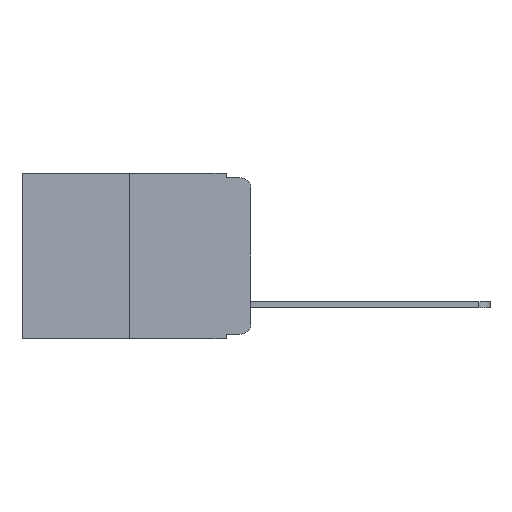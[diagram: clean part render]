
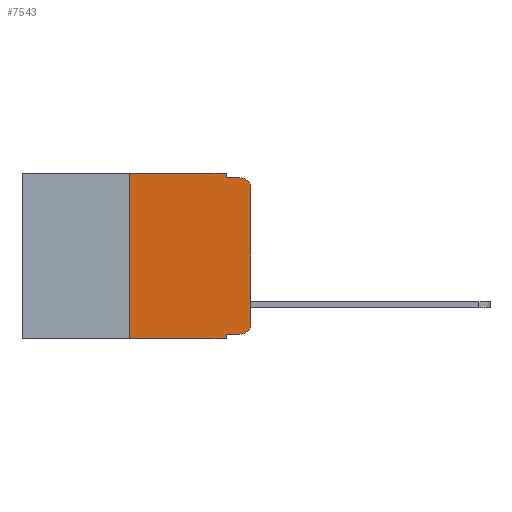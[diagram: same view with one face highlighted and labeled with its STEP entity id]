
A CAD part, left-side view. The second image highlights one B-rep face of the part: STEP entity #7543.
In plain terms, the highlighted planar face has unit normal (-1, 0, 0).
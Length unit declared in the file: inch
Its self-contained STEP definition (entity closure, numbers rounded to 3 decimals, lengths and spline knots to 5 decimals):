
#147 = CARTESIAN_POINT ( 'NONE',  ( 0., 0.051, -0.01 ) ) ;
#233 = VERTEX_POINT ( 'NONE', #2230 ) ;
#264 = FACE_OUTER_BOUND ( 'NONE', #621, .T. ) ;
#532 = EDGE_CURVE ( 'NONE', #1298, #7820, #5240, .T. ) ;
#621 = EDGE_LOOP ( 'NONE', ( #12457, #2009, #9173, #11586, #6703, #9820, #10135, #4715, #13458, #6718 ) ) ;
#705 = CARTESIAN_POINT ( 'NONE',  ( 0., 0.051, -0.01 ) ) ;
#788 = CARTESIAN_POINT ( 'NONE',  ( 0., 0.02, -0.03 ) ) ;
#1298 = VERTEX_POINT ( 'NONE', #6933 ) ;
#1445 = EDGE_CURVE ( 'NONE', #3596, #2863, #10079, .T. ) ;
#1558 = VERTEX_POINT ( 'NONE', #705 ) ;
#2009 = ORIENTED_EDGE ( 'NONE', *, *, #5065, .T. ) ;
#2223 = CARTESIAN_POINT ( 'NONE',  ( 0., 0.473, 0. ) ) ;
#2230 = CARTESIAN_POINT ( 'NONE',  ( 0., 0.051, -0.333 ) ) ;
#2386 = CARTESIAN_POINT ( 'NONE',  ( 0., 0., -0.313 ) ) ;
#2401 = LINE ( 'NONE', #6328, #5292 ) ;
#2863 = VERTEX_POINT ( 'NONE', #5200 ) ;
#3043 = VECTOR ( 'NONE', #9039, 39.37008 ) ;
#3350 = DIRECTION ( 'NONE',  ( 0., 0., -1. ) ) ;
#3360 = VECTOR ( 'NONE', #6534, 39.37008 ) ;
#3596 = VERTEX_POINT ( 'NONE', #11153 ) ;
#3992 = PLANE ( 'NONE',  #8873 ) ;
#4229 = VERTEX_POINT ( 'NONE', #9750 ) ;
#4387 = EDGE_CURVE ( 'NONE', #233, #1298, #12742, .T. ) ;
#4494 = EDGE_CURVE ( 'NONE', #233, #2863, #8756, .T. ) ;
#4715 = ORIENTED_EDGE ( 'NONE', *, *, #4494, .F. ) ;
#4903 = EDGE_CURVE ( 'NONE', #3596, #4229, #2401, .T. ) ;
#4940 = DIRECTION ( 'NONE',  ( 0., 0., 1. ) ) ;
#4987 = EDGE_CURVE ( 'NONE', #13226, #1558, #10303, .T. ) ;
#5034 = EDGE_CURVE ( 'NONE', #1558, #12018, #10771, .T. ) ;
#5065 = EDGE_CURVE ( 'NONE', #11620, #12018, #12674, .T. ) ;
#5070 = EDGE_CURVE ( 'NONE', #7820, #11620, #8205, .T. ) ;
#5192 = CARTESIAN_POINT ( 'NONE',  ( 0., 0.051, -0.333 ) ) ;
#5200 = CARTESIAN_POINT ( 'NONE',  ( 0., 0.051, -0.343 ) ) ;
#5240 = CIRCLE ( 'NONE', #11673, 0.02 ) ;
#5292 = VECTOR ( 'NONE', #12916, 39.37008 ) ;
#5376 = DIRECTION ( 'NONE',  ( 0., -1., 0. ) ) ;
#5501 = CARTESIAN_POINT ( 'NONE',  ( 0., 0.02, -0.01 ) ) ;
#5627 = DIRECTION ( 'NONE',  ( 0., -1., 0. ) ) ;
#6017 = AXIS2_PLACEMENT_3D ( 'NONE', #788, #8937, #8815 ) ;
#6307 = EDGE_CURVE ( 'NONE', #4229, #13226, #9093, .T. ) ;
#6328 = CARTESIAN_POINT ( 'NONE',  ( 0., 0.25, 0. ) ) ;
#6420 = DIRECTION ( 'NONE',  ( 1., 0., 0. ) ) ;
#6534 = DIRECTION ( 'NONE',  ( 0., 0., -1. ) ) ;
#6703 = ORIENTED_EDGE ( 'NONE', *, *, #6307, .F. ) ;
#6718 = ORIENTED_EDGE ( 'NONE', *, *, #532, .T. ) ;
#6933 = CARTESIAN_POINT ( 'NONE',  ( 0., 0.02, -0.333 ) ) ;
#7212 = VECTOR ( 'NONE', #3350, 39.37008 ) ;
#7455 = CARTESIAN_POINT ( 'NONE',  ( 0., 0.473, 0. ) ) ;
#7491 = VECTOR ( 'NONE', #4940, 39.37008 ) ;
#7543 = ADVANCED_FACE ( 'NONE', ( #264 ), #3992, .F. ) ;
#7820 = VERTEX_POINT ( 'NONE', #2386 ) ;
#8205 = LINE ( 'NONE', #11141, #7491 ) ;
#8287 = VECTOR ( 'NONE', #5376, 39.37008 ) ;
#8756 = LINE ( 'NONE', #12577, #3360 ) ;
#8815 = DIRECTION ( 'NONE',  ( 0., 0., -1. ) ) ;
#8873 = AXIS2_PLACEMENT_3D ( 'NONE', #7455, #6420, #12978 ) ;
#8884 = CARTESIAN_POINT ( 'NONE',  ( 0., 0.051, 0. ) ) ;
#8937 = DIRECTION ( 'NONE',  ( -1., 0., 0. ) ) ;
#9039 = DIRECTION ( 'NONE',  ( 0., -1., 0. ) ) ;
#9093 = LINE ( 'NONE', #2223, #3043 ) ;
#9145 = DIRECTION ( 'NONE',  ( 0., -1., 0. ) ) ;
#9173 = ORIENTED_EDGE ( 'NONE', *, *, #5034, .F. ) ;
#9418 = CARTESIAN_POINT ( 'NONE',  ( 0., 0.051, 0. ) ) ;
#9750 = CARTESIAN_POINT ( 'NONE',  ( 0., 0.25, 0. ) ) ;
#9820 = ORIENTED_EDGE ( 'NONE', *, *, #4903, .F. ) ;
#9930 = DIRECTION ( 'NONE',  ( 0., 0., -1. ) ) ;
#10079 = LINE ( 'NONE', #10594, #12043 ) ;
#10135 = ORIENTED_EDGE ( 'NONE', *, *, #1445, .T. ) ;
#10303 = LINE ( 'NONE', #9418, #7212 ) ;
#10594 = CARTESIAN_POINT ( 'NONE',  ( 0., 0.473, -0.343 ) ) ;
#10771 = LINE ( 'NONE', #147, #12932 ) ;
#11141 = CARTESIAN_POINT ( 'NONE',  ( 0., 0., 0. ) ) ;
#11153 = CARTESIAN_POINT ( 'NONE',  ( 0., 0.25, -0.343 ) ) ;
#11586 = ORIENTED_EDGE ( 'NONE', *, *, #4987, .F. ) ;
#11620 = VERTEX_POINT ( 'NONE', #12184 ) ;
#11673 = AXIS2_PLACEMENT_3D ( 'NONE', #12491, #12684, #9930 ) ;
#12018 = VERTEX_POINT ( 'NONE', #5501 ) ;
#12043 = VECTOR ( 'NONE', #9145, 39.37008 ) ;
#12184 = CARTESIAN_POINT ( 'NONE',  ( 0., 0., -0.03 ) ) ;
#12457 = ORIENTED_EDGE ( 'NONE', *, *, #5070, .T. ) ;
#12491 = CARTESIAN_POINT ( 'NONE',  ( 0., 0.02, -0.313 ) ) ;
#12577 = CARTESIAN_POINT ( 'NONE',  ( 0., 0.051, 0. ) ) ;
#12674 = CIRCLE ( 'NONE', #6017, 0.02 ) ;
#12684 = DIRECTION ( 'NONE',  ( -1., 0., 0. ) ) ;
#12742 = LINE ( 'NONE', #5192, #8287 ) ;
#12916 = DIRECTION ( 'NONE',  ( 0., 0., 1. ) ) ;
#12932 = VECTOR ( 'NONE', #5627, 39.37008 ) ;
#12978 = DIRECTION ( 'NONE',  ( 0., 0., -1. ) ) ;
#13226 = VERTEX_POINT ( 'NONE', #8884 ) ;
#13458 = ORIENTED_EDGE ( 'NONE', *, *, #4387, .T. ) ;
